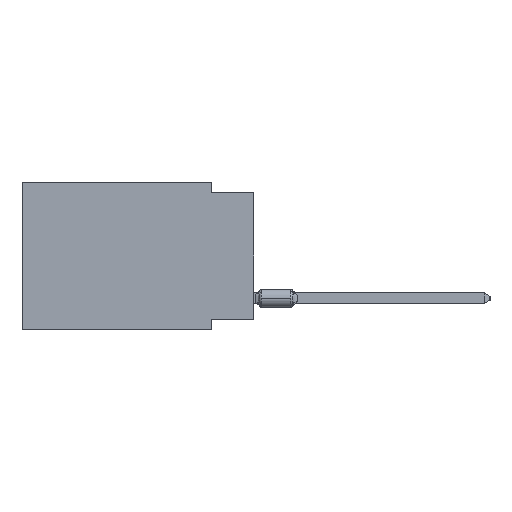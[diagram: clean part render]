
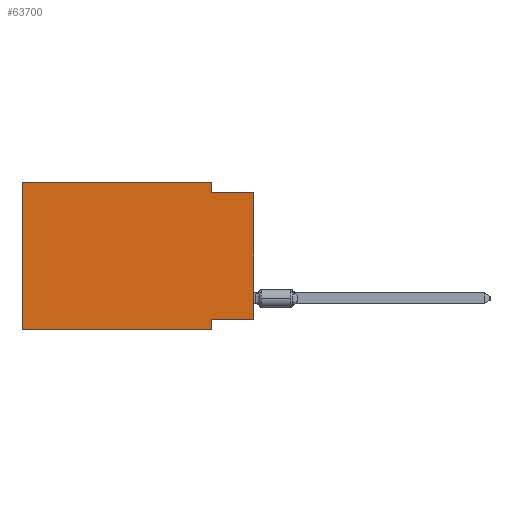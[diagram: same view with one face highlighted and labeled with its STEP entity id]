
A CAD part, left-side view. The second image highlights one B-rep face of the part: STEP entity #63700.
In plain terms, the highlighted planar face has unit normal (-1, 0, 0).
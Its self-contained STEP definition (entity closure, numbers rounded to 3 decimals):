
#856 = CARTESIAN_POINT ( 'NONE',  ( 0., 2.54, 0. ) ) ;
#924 = ORIENTED_EDGE ( 'NONE', *, *, #32316, .F. ) ;
#948 = LINE ( 'NONE', #61383, #91576 ) ;
#6208 = PLANE ( 'NONE',  #82506 ) ;
#6699 = DIRECTION ( 'NONE',  ( 1., 0., 0. ) ) ;
#8760 = ORIENTED_EDGE ( 'NONE', *, *, #53359, .T. ) ;
#9769 = EDGE_LOOP ( 'NONE', ( #8760, #87075, #40737, #11914, #924, #87931, #93124, #72388 ) ) ;
#9870 = VERTEX_POINT ( 'NONE', #40490 ) ;
#11765 = DIRECTION ( 'NONE',  ( 0., 0., -1. ) ) ;
#11914 = ORIENTED_EDGE ( 'NONE', *, *, #74698, .F. ) ;
#17106 = VERTEX_POINT ( 'NONE', #86711 ) ;
#18151 = DIRECTION ( 'NONE',  ( 0., 1., 0. ) ) ;
#20365 = VECTOR ( 'NONE', #47016, 1000. ) ;
#23643 = DIRECTION ( 'NONE',  ( 0., 0., 1. ) ) ;
#24367 = CARTESIAN_POINT ( 'NONE',  ( 0., 2.54, -8.89 ) ) ;
#26120 = VERTEX_POINT ( 'NONE', #99220 ) ;
#26445 = VERTEX_POINT ( 'NONE', #856 ) ;
#26927 = VERTEX_POINT ( 'NONE', #95609 ) ;
#28083 = VECTOR ( 'NONE', #18151, 1000. ) ;
#29976 = DIRECTION ( 'NONE',  ( 0., -1., 0. ) ) ;
#32316 = EDGE_CURVE ( 'NONE', #17106, #26927, #87069, .T. ) ;
#33115 = EDGE_CURVE ( 'NONE', #9870, #26120, #72534, .T. ) ;
#36281 = VECTOR ( 'NONE', #37184, 1000. ) ;
#37125 = VERTEX_POINT ( 'NONE', #71414 ) ;
#37184 = DIRECTION ( 'NONE',  ( 0., 0., 1. ) ) ;
#37817 = LINE ( 'NONE', #45875, #82212 ) ;
#38541 = CARTESIAN_POINT ( 'NONE',  ( 0., 0., -0.635 ) ) ;
#40490 = CARTESIAN_POINT ( 'NONE',  ( 0., 0., -8.255 ) ) ;
#40737 = ORIENTED_EDGE ( 'NONE', *, *, #61459, .F. ) ;
#43480 = CARTESIAN_POINT ( 'NONE',  ( 0., 2.54, 0. ) ) ;
#45034 = CARTESIAN_POINT ( 'NONE',  ( 0., 2.54, -8.89 ) ) ;
#45875 = CARTESIAN_POINT ( 'NONE',  ( 0., 13.97, -8.89 ) ) ;
#47016 = DIRECTION ( 'NONE',  ( 0., 0., -1. ) ) ;
#48039 = EDGE_CURVE ( 'NONE', #17106, #81828, #37817, .T. ) ;
#53359 = EDGE_CURVE ( 'NONE', #9870, #37125, #99149, .T. ) ;
#58595 = CARTESIAN_POINT ( 'NONE',  ( 0., 13.97, 0. ) ) ;
#59099 = FACE_OUTER_BOUND ( 'NONE', #9769, .T. ) ;
#59860 = CARTESIAN_POINT ( 'NONE',  ( 0., 0., 0. ) ) ;
#61383 = CARTESIAN_POINT ( 'NONE',  ( 0., 13.97, 0. ) ) ;
#61459 = EDGE_CURVE ( 'NONE', #26445, #79298, #74692, .T. ) ;
#63700 = ADVANCED_FACE ( 'NONE', ( #59099 ), #6208, .F. ) ;
#65555 = EDGE_CURVE ( 'NONE', #26120, #81828, #99459, .T. ) ;
#69970 = VECTOR ( 'NONE', #29976, 1000. ) ;
#71414 = CARTESIAN_POINT ( 'NONE',  ( 0., 0., -0.635 ) ) ;
#72388 = ORIENTED_EDGE ( 'NONE', *, *, #33115, .F. ) ;
#72534 = LINE ( 'NONE', #73024, #28083 ) ;
#73024 = CARTESIAN_POINT ( 'NONE',  ( 0., 0., -8.255 ) ) ;
#74107 = VECTOR ( 'NONE', #11765, 1000. ) ;
#74692 = LINE ( 'NONE', #43480, #74107 ) ;
#74698 = EDGE_CURVE ( 'NONE', #26927, #26445, #948, .T. ) ;
#77501 = CARTESIAN_POINT ( 'NONE',  ( 0., 13.97, 0. ) ) ;
#79298 = VERTEX_POINT ( 'NONE', #96061 ) ;
#81828 = VERTEX_POINT ( 'NONE', #45034 ) ;
#82212 = VECTOR ( 'NONE', #91726, 1000. ) ;
#82506 = AXIS2_PLACEMENT_3D ( 'NONE', #58595, #6699, #89823 ) ;
#85062 = DIRECTION ( 'NONE',  ( 0., -1., 0. ) ) ;
#86711 = CARTESIAN_POINT ( 'NONE',  ( 0., 13.97, -8.89 ) ) ;
#87069 = LINE ( 'NONE', #77501, #93974 ) ;
#87075 = ORIENTED_EDGE ( 'NONE', *, *, #93388, .F. ) ;
#87931 = ORIENTED_EDGE ( 'NONE', *, *, #48039, .T. ) ;
#89823 = DIRECTION ( 'NONE',  ( 0., 0., -1. ) ) ;
#91576 = VECTOR ( 'NONE', #85062, 1000. ) ;
#91726 = DIRECTION ( 'NONE',  ( 0., -1., 0. ) ) ;
#93124 = ORIENTED_EDGE ( 'NONE', *, *, #65555, .F. ) ;
#93388 = EDGE_CURVE ( 'NONE', #79298, #37125, #98999, .T. ) ;
#93974 = VECTOR ( 'NONE', #23643, 1000. ) ;
#95609 = CARTESIAN_POINT ( 'NONE',  ( 0., 13.97, 0. ) ) ;
#96061 = CARTESIAN_POINT ( 'NONE',  ( 0., 2.54, -0.635 ) ) ;
#98999 = LINE ( 'NONE', #38541, #69970 ) ;
#99149 = LINE ( 'NONE', #59860, #36281 ) ;
#99220 = CARTESIAN_POINT ( 'NONE',  ( 0., 2.54, -8.255 ) ) ;
#99459 = LINE ( 'NONE', #24367, #20365 ) ;
